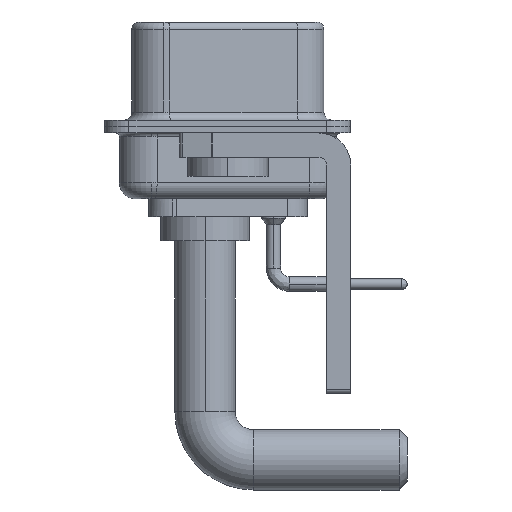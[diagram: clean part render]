
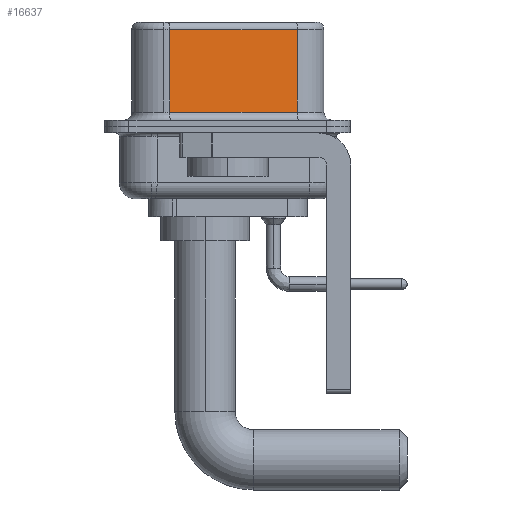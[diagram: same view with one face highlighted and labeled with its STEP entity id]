
A CAD part, left-side view. The second image highlights one B-rep face of the part: STEP entity #16637.
In plain terms, the highlighted planar face has unit normal (-0.985, -0.174, 0).
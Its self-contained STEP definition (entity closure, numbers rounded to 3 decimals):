
#56 = ORIENTED_EDGE ( 'NONE', *, *, #11801, .T. ) ;
#750 = VECTOR ( 'NONE', #13751, 1000. ) ;
#3277 = ORIENTED_EDGE ( 'NONE', *, *, #20165, .T. ) ;
#3375 = DIRECTION ( 'NONE',  ( -0.174, 0.985, 0. ) ) ;
#4302 = CARTESIAN_POINT ( 'NONE',  ( 3.73, 3.628, 6.52 ) ) ;
#4703 = LINE ( 'NONE', #24169, #4842 ) ;
#4842 = VECTOR ( 'NONE', #14159, 1000. ) ;
#4863 = EDGE_CURVE ( 'NONE', #20966, #9038, #17311, .T. ) ;
#6952 = CARTESIAN_POINT ( 'NONE',  ( 5.132, -4.322, 6.52 ) ) ;
#7364 = ORIENTED_EDGE ( 'NONE', *, *, #4863, .F. ) ;
#8355 = EDGE_CURVE ( 'NONE', #20664, #8369, #19760, .T. ) ;
#8369 = VERTEX_POINT ( 'NONE', #20239 ) ;
#8550 = VECTOR ( 'NONE', #3375, 1000. ) ;
#8633 = VECTOR ( 'NONE', #17550, 1000. ) ;
#9038 = VERTEX_POINT ( 'NONE', #18829 ) ;
#10716 = EDGE_LOOP ( 'NONE', ( #7364, #3277, #19886, #56 ) ) ;
#11801 = EDGE_CURVE ( 'NONE', #8369, #9038, #4703, .T. ) ;
#12451 = LINE ( 'NONE', #14345, #8550 ) ;
#13751 = DIRECTION ( 'NONE',  ( 0., 0., -1. ) ) ;
#14159 = DIRECTION ( 'NONE',  ( 0.174, -0.985, 0. ) ) ;
#14345 = CARTESIAN_POINT ( 'NONE',  ( 5.132, -4.322, 6.02 ) ) ;
#14518 = PLANE ( 'NONE',  #14519 ) ;
#14519 = AXIS2_PLACEMENT_3D ( 'NONE', #6952, #14644, #22522 ) ;
#14644 = DIRECTION ( 'NONE',  ( 0.985, 0.174, 0. ) ) ;
#16637 = ADVANCED_FACE ( 'NONE', ( #24162 ), #14518, .F. ) ;
#17311 = LINE ( 'NONE', #23072, #8633 ) ;
#17550 = DIRECTION ( 'NONE',  ( 0., 0., -1. ) ) ;
#18043 = CARTESIAN_POINT ( 'NONE',  ( 3.73, 3.628, 6.02 ) ) ;
#18829 = CARTESIAN_POINT ( 'NONE',  ( 5.132, -4.322, 0.9 ) ) ;
#19148 = CARTESIAN_POINT ( 'NONE',  ( 5.132, -4.322, 6.02 ) ) ;
#19760 = LINE ( 'NONE', #4302, #750 ) ;
#19886 = ORIENTED_EDGE ( 'NONE', *, *, #8355, .T. ) ;
#20165 = EDGE_CURVE ( 'NONE', #20966, #20664, #12451, .T. ) ;
#20239 = CARTESIAN_POINT ( 'NONE',  ( 3.73, 3.628, 0.9 ) ) ;
#20664 = VERTEX_POINT ( 'NONE', #18043 ) ;
#20966 = VERTEX_POINT ( 'NONE', #19148 ) ;
#22522 = DIRECTION ( 'NONE',  ( -0.174, 0.985, 0. ) ) ;
#23072 = CARTESIAN_POINT ( 'NONE',  ( 5.132, -4.322, 6.52 ) ) ;
#24162 = FACE_OUTER_BOUND ( 'NONE', #10716, .T. ) ;
#24169 = CARTESIAN_POINT ( 'NONE',  ( 5.132, -4.322, 0.9 ) ) ;
